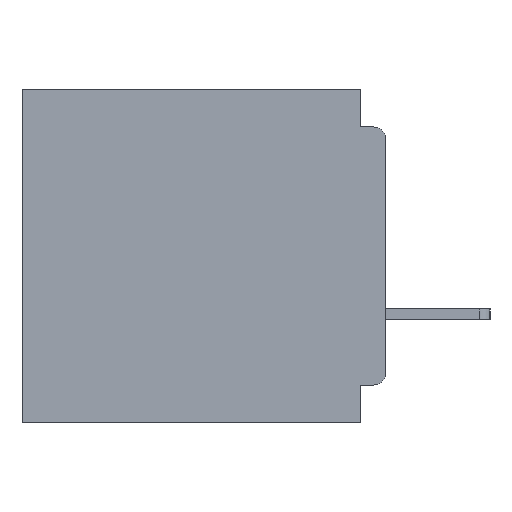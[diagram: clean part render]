
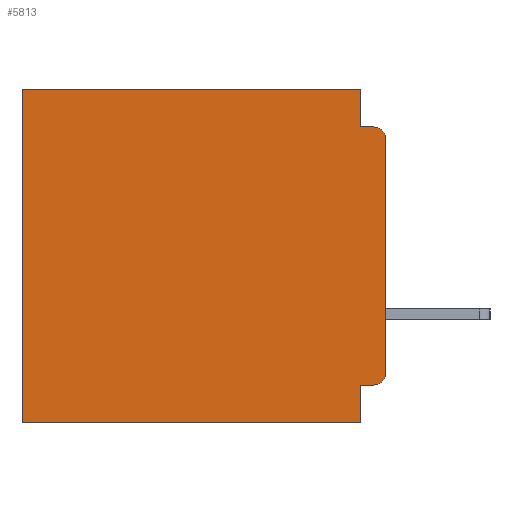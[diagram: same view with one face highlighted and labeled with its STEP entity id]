
A CAD part, left-side view. The second image highlights one B-rep face of the part: STEP entity #5813.
In plain terms, the highlighted planar face has unit normal (-1, 0, 0).
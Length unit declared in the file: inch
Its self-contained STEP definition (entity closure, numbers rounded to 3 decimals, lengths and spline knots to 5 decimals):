
#28 = CARTESIAN_POINT ( 'NONE',  ( 0.3, 0.015, -0.045 ) ) ;
#350 = DIRECTION ( 'NONE',  ( 0., -1., 0. ) ) ;
#741 = CARTESIAN_POINT ( 'NONE',  ( 0.3, 0.437, -0.4 ) ) ;
#918 = VECTOR ( 'NONE', #350, 39.37008 ) ;
#2360 = VECTOR ( 'NONE', #12714, 39.37008 ) ;
#2453 = ORIENTED_EDGE ( 'NONE', *, *, #41035, .T. ) ;
#2842 = ORIENTED_EDGE ( 'NONE', *, *, #4277, .F. ) ;
#2855 = PLANE ( 'NONE',  #14748 ) ;
#2915 = AXIS2_PLACEMENT_3D ( 'NONE', #32676, #12881, #35974 ) ;
#2942 = CARTESIAN_POINT ( 'NONE',  ( 0.3, 0.031, 0. ) ) ;
#3759 = CARTESIAN_POINT ( 'NONE',  ( 0.3, 0., -0.045 ) ) ;
#3909 = CARTESIAN_POINT ( 'NONE',  ( 0.3, 0., -0.06 ) ) ;
#4277 = EDGE_CURVE ( 'NONE', #37430, #12170, #18734, .T. ) ;
#5539 = CARTESIAN_POINT ( 'NONE',  ( 0.3, 0., -0.4 ) ) ;
#5813 = ADVANCED_FACE ( 'NONE', ( #25829 ), #2855, .F. ) ;
#6229 = DIRECTION ( 'NONE',  ( 1., 0., 0. ) ) ;
#7874 = DIRECTION ( 'NONE',  ( 0., 1., 0. ) ) ;
#7932 = CARTESIAN_POINT ( 'NONE',  ( 0.3, 0.031, -0.045 ) ) ;
#8353 = CARTESIAN_POINT ( 'NONE',  ( 0.3, 0.437, 0. ) ) ;
#9410 = EDGE_CURVE ( 'NONE', #23599, #24703, #31734, .T. ) ;
#9772 = CIRCLE ( 'NONE', #2915, 0.015 ) ;
#10276 = ORIENTED_EDGE ( 'NONE', *, *, #14346, .F. ) ;
#12170 = VERTEX_POINT ( 'NONE', #30901 ) ;
#12662 = LINE ( 'NONE', #741, #18380 ) ;
#12714 = DIRECTION ( 'NONE',  ( 0., 0., -1. ) ) ;
#12881 = DIRECTION ( 'NONE',  ( -1., 0., 0. ) ) ;
#13037 = CARTESIAN_POINT ( 'NONE',  ( 0.3, 0.015, -0.06 ) ) ;
#13148 = VERTEX_POINT ( 'NONE', #42549 ) ;
#14346 = EDGE_CURVE ( 'NONE', #24703, #37430, #40201, .T. ) ;
#14748 = AXIS2_PLACEMENT_3D ( 'NONE', #39180, #6229, #29511 ) ;
#15529 = LINE ( 'NONE', #19479, #40736 ) ;
#15787 = ORIENTED_EDGE ( 'NONE', *, *, #40019, .F. ) ;
#15863 = ORIENTED_EDGE ( 'NONE', *, *, #9410, .F. ) ;
#16373 = DIRECTION ( 'NONE',  ( 0., 0., -1. ) ) ;
#17603 = DIRECTION ( 'NONE',  ( 0., 0., -1. ) ) ;
#18380 = VECTOR ( 'NONE', #17603, 39.37008 ) ;
#18383 = VERTEX_POINT ( 'NONE', #23460 ) ;
#18484 = VERTEX_POINT ( 'NONE', #3909 ) ;
#18734 = LINE ( 'NONE', #5539, #35202 ) ;
#18750 = LINE ( 'NONE', #3759, #918 ) ;
#19108 = EDGE_CURVE ( 'NONE', #29288, #12170, #12662, .T. ) ;
#19479 = CARTESIAN_POINT ( 'NONE',  ( 0.3, 0., 0. ) ) ;
#21677 = VECTOR ( 'NONE', #32718, 39.37008 ) ;
#21957 = VECTOR ( 'NONE', #7874, 39.37008 ) ;
#22774 = VECTOR ( 'NONE', #42879, 39.37008 ) ;
#22801 = DIRECTION ( 'NONE',  ( 0., 1., 0. ) ) ;
#22975 = VERTEX_POINT ( 'NONE', #28 ) ;
#23292 = CARTESIAN_POINT ( 'NONE',  ( 0.3, 0.031, -0.4 ) ) ;
#23384 = CARTESIAN_POINT ( 'NONE',  ( 0.3, 0.015, -0.355 ) ) ;
#23460 = CARTESIAN_POINT ( 'NONE',  ( 0.3, 0.031, 0. ) ) ;
#23561 = ORIENTED_EDGE ( 'NONE', *, *, #24104, .T. ) ;
#23599 = VERTEX_POINT ( 'NONE', #23384 ) ;
#24104 = EDGE_CURVE ( 'NONE', #23599, #13148, #9772, .T. ) ;
#24494 = CARTESIAN_POINT ( 'NONE',  ( 0.3, 0., -0.355 ) ) ;
#24703 = VERTEX_POINT ( 'NONE', #38132 ) ;
#25829 = FACE_OUTER_BOUND ( 'NONE', #37990, .T. ) ;
#27325 = VERTEX_POINT ( 'NONE', #7932 ) ;
#28708 = CARTESIAN_POINT ( 'NONE',  ( 0.3, 0.031, -0.4 ) ) ;
#29288 = VERTEX_POINT ( 'NONE', #8353 ) ;
#29511 = DIRECTION ( 'NONE',  ( 0., 0., -1. ) ) ;
#30194 = ORIENTED_EDGE ( 'NONE', *, *, #19108, .T. ) ;
#30462 = LINE ( 'NONE', #2942, #21677 ) ;
#30901 = CARTESIAN_POINT ( 'NONE',  ( 0.3, 0.437, -0.4 ) ) ;
#30920 = ORIENTED_EDGE ( 'NONE', *, *, #35811, .F. ) ;
#31734 = LINE ( 'NONE', #24494, #21957 ) ;
#32676 = CARTESIAN_POINT ( 'NONE',  ( 0.3, 0.015, -0.34 ) ) ;
#32718 = DIRECTION ( 'NONE',  ( 0., 0., -1. ) ) ;
#32991 = AXIS2_PLACEMENT_3D ( 'NONE', #13037, #36105, #16373 ) ;
#33554 = ORIENTED_EDGE ( 'NONE', *, *, #40937, .T. ) ;
#35202 = VECTOR ( 'NONE', #35781, 39.37008 ) ;
#35781 = DIRECTION ( 'NONE',  ( 0., 1., 0. ) ) ;
#35798 = CARTESIAN_POINT ( 'NONE',  ( 0.3, 0., -0.4 ) ) ;
#35811 = EDGE_CURVE ( 'NONE', #18383, #27325, #30462, .T. ) ;
#35974 = DIRECTION ( 'NONE',  ( 0., 0., -1. ) ) ;
#36105 = DIRECTION ( 'NONE',  ( -1., 0., 0. ) ) ;
#37430 = VERTEX_POINT ( 'NONE', #28708 ) ;
#37633 = LINE ( 'NONE', #35798, #2360 ) ;
#37670 = CIRCLE ( 'NONE', #32991, 0.015 ) ;
#37990 = EDGE_LOOP ( 'NONE', ( #41205, #2453, #15787, #30920, #33554, #30194, #2842, #10276, #15863, #23561 ) ) ;
#38132 = CARTESIAN_POINT ( 'NONE',  ( 0.3, 0.031, -0.355 ) ) ;
#39180 = CARTESIAN_POINT ( 'NONE',  ( 0.3, 0., -0.4 ) ) ;
#40019 = EDGE_CURVE ( 'NONE', #27325, #22975, #18750, .T. ) ;
#40201 = LINE ( 'NONE', #23292, #22774 ) ;
#40736 = VECTOR ( 'NONE', #22801, 39.37008 ) ;
#40937 = EDGE_CURVE ( 'NONE', #18383, #29288, #15529, .T. ) ;
#41035 = EDGE_CURVE ( 'NONE', #18484, #22975, #37670, .T. ) ;
#41205 = ORIENTED_EDGE ( 'NONE', *, *, #41480, .F. ) ;
#41480 = EDGE_CURVE ( 'NONE', #18484, #13148, #37633, .T. ) ;
#42549 = CARTESIAN_POINT ( 'NONE',  ( 0.3, 0., -0.34 ) ) ;
#42879 = DIRECTION ( 'NONE',  ( 0., 0., -1. ) ) ;
